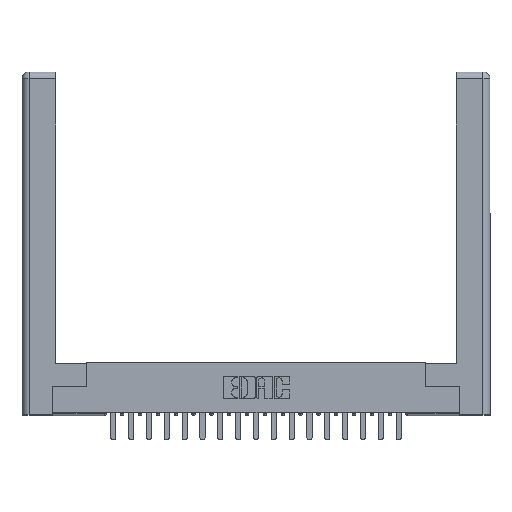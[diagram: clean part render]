
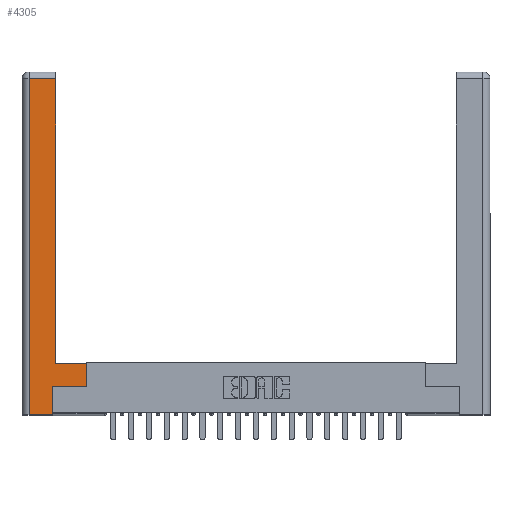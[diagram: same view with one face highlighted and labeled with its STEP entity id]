
A CAD part, top view. The second image highlights one B-rep face of the part: STEP entity #4305.
In plain terms, the highlighted planar face has unit normal (0, 0, 1).
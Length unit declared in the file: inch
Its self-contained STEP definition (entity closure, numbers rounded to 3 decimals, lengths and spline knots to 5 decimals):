
#443 = LINE ( 'NONE', #2069, #19226 ) ;
#453 = VECTOR ( 'NONE', #8641, 39.37008 ) ;
#524 = LINE ( 'NONE', #21478, #14680 ) ;
#2069 = CARTESIAN_POINT ( 'NONE',  ( 0.0615, 2.94, 0. ) ) ;
#2226 = VECTOR ( 'NONE', #10540, 39.37008 ) ;
#3215 = VERTEX_POINT ( 'NONE', #19051 ) ;
#3363 = CARTESIAN_POINT ( 'NONE',  ( 0.295, 2.94, 0. ) ) ;
#3577 = LINE ( 'NONE', #21817, #14584 ) ;
#3869 = DIRECTION ( 'NONE',  ( 0., 0., -1. ) ) ;
#3950 = VERTEX_POINT ( 'NONE', #15498 ) ;
#3957 = LINE ( 'NONE', #8293, #2226 ) ;
#4095 = PLANE ( 'NONE',  #7305 ) ;
#4305 = ADVANCED_FACE ( 'NONE', ( #14721 ), #4095, .F. ) ;
#4575 = VERTEX_POINT ( 'NONE', #3363 ) ;
#5000 = EDGE_CURVE ( 'NONE', #3215, #3950, #14095, .T. ) ;
#5116 = DIRECTION ( 'NONE',  ( 0., 1., 0. ) ) ;
#5149 = EDGE_CURVE ( 'NONE', #23851, #19892, #524, .T. ) ;
#5542 = EDGE_LOOP ( 'NONE', ( #6062, #12429, #13191, #12913, #14098, #12409, #19069, #11621 ) ) ;
#5594 = VERTEX_POINT ( 'NONE', #22150 ) ;
#5983 = CARTESIAN_POINT ( 'NONE',  ( 0.295, 3., 0. ) ) ;
#6062 = ORIENTED_EDGE ( 'NONE', *, *, #23232, .T. ) ;
#7305 = AXIS2_PLACEMENT_3D ( 'NONE', #9378, #3869, #15048 ) ;
#8293 = CARTESIAN_POINT ( 'NONE',  ( 0.565, 0.45, 0. ) ) ;
#8641 = DIRECTION ( 'NONE',  ( 1., 0., 0. ) ) ;
#8957 = EDGE_CURVE ( 'NONE', #4575, #23851, #443, .T. ) ;
#9270 = CARTESIAN_POINT ( 'NONE',  ( 0.265, 0., 0. ) ) ;
#9378 = CARTESIAN_POINT ( 'NONE',  ( 0., 0., 0. ) ) ;
#9892 = CARTESIAN_POINT ( 'NONE',  ( 0.565, 0.245, 0. ) ) ;
#10540 = DIRECTION ( 'NONE',  ( 0., 1., 0. ) ) ;
#11621 = ORIENTED_EDGE ( 'NONE', *, *, #16185, .T. ) ;
#11693 = VERTEX_POINT ( 'NONE', #9270 ) ;
#12232 = CARTESIAN_POINT ( 'NONE',  ( 0.565, 0.45, 0. ) ) ;
#12409 = ORIENTED_EDGE ( 'NONE', *, *, #5000, .T. ) ;
#12429 = ORIENTED_EDGE ( 'NONE', *, *, #8957, .T. ) ;
#12586 = LINE ( 'NONE', #23481, #453 ) ;
#12913 = ORIENTED_EDGE ( 'NONE', *, *, #17630, .T. ) ;
#13191 = ORIENTED_EDGE ( 'NONE', *, *, #5149, .T. ) ;
#13234 = VECTOR ( 'NONE', #21854, 39.37008 ) ;
#13691 = CARTESIAN_POINT ( 'NONE',  ( 0.0615, 0., 0. ) ) ;
#13697 = DIRECTION ( 'NONE',  ( 1., 0., 0. ) ) ;
#14095 = LINE ( 'NONE', #9892, #18141 ) ;
#14098 = ORIENTED_EDGE ( 'NONE', *, *, #21599, .T. ) ;
#14584 = VECTOR ( 'NONE', #5116, 39.37008 ) ;
#14680 = VECTOR ( 'NONE', #19672, 39.37008 ) ;
#14721 = FACE_OUTER_BOUND ( 'NONE', #5542, .T. ) ;
#15048 = DIRECTION ( 'NONE',  ( -1., 0., 0. ) ) ;
#15498 = CARTESIAN_POINT ( 'NONE',  ( 0.565, 0.245, 0. ) ) ;
#16185 = EDGE_CURVE ( 'NONE', #18023, #5594, #21354, .T. ) ;
#17630 = EDGE_CURVE ( 'NONE', #19892, #11693, #12586, .T. ) ;
#18023 = VERTEX_POINT ( 'NONE', #12232 ) ;
#18141 = VECTOR ( 'NONE', #13697, 39.37008 ) ;
#18583 = LINE ( 'NONE', #5983, #22374 ) ;
#18709 = DIRECTION ( 'NONE',  ( -1., 0., 0. ) ) ;
#19051 = CARTESIAN_POINT ( 'NONE',  ( 0.265, 0.245, 0. ) ) ;
#19069 = ORIENTED_EDGE ( 'NONE', *, *, #20486, .T. ) ;
#19226 = VECTOR ( 'NONE', #18709, 39.37008 ) ;
#19672 = DIRECTION ( 'NONE',  ( 0., -1., 0. ) ) ;
#19892 = VERTEX_POINT ( 'NONE', #13691 ) ;
#20048 = CARTESIAN_POINT ( 'NONE',  ( 0.295, 0.45, 0. ) ) ;
#20486 = EDGE_CURVE ( 'NONE', #3950, #18023, #3957, .T. ) ;
#21158 = CARTESIAN_POINT ( 'NONE',  ( 0.0615, 2.94, 0. ) ) ;
#21354 = LINE ( 'NONE', #20048, #13234 ) ;
#21478 = CARTESIAN_POINT ( 'NONE',  ( 0.0615, 0., 0. ) ) ;
#21599 = EDGE_CURVE ( 'NONE', #11693, #3215, #3577, .T. ) ;
#21817 = CARTESIAN_POINT ( 'NONE',  ( 0.265, 0.245, 0. ) ) ;
#21854 = DIRECTION ( 'NONE',  ( -1., 0., 0. ) ) ;
#22150 = CARTESIAN_POINT ( 'NONE',  ( 0.295, 0.45, 0. ) ) ;
#22374 = VECTOR ( 'NONE', #22619, 39.37008 ) ;
#22619 = DIRECTION ( 'NONE',  ( 0., 1., 0. ) ) ;
#23232 = EDGE_CURVE ( 'NONE', #5594, #4575, #18583, .T. ) ;
#23481 = CARTESIAN_POINT ( 'NONE',  ( 0.265, 0., 0. ) ) ;
#23851 = VERTEX_POINT ( 'NONE', #21158 ) ;
